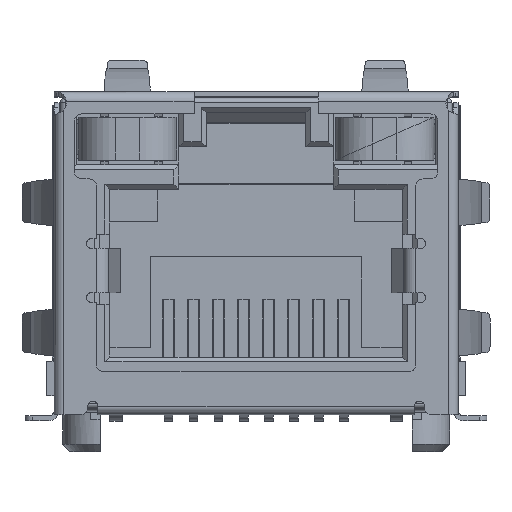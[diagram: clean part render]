
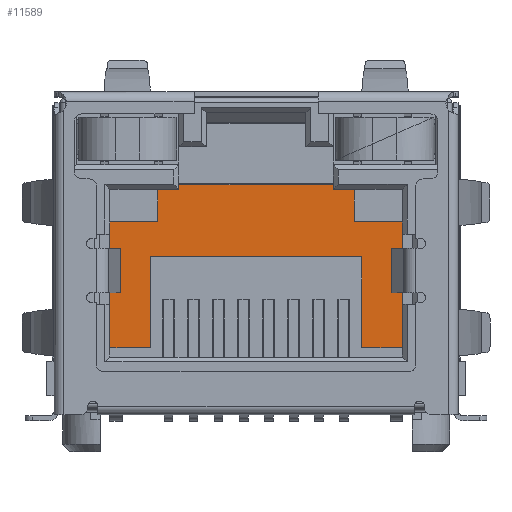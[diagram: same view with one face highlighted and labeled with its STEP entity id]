
A CAD part, top view. The second image highlights one B-rep face of the part: STEP entity #11589.
In plain terms, the highlighted planar face has unit normal (0, 0, 1).
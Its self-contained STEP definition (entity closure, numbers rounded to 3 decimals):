
#21 = LINE ( 'NONE', #16234, #8757 ) ;
#443 = CARTESIAN_POINT ( 'NONE',  ( 12.275, 2.65, -12. ) ) ;
#582 = ORIENTED_EDGE ( 'NONE', *, *, #8021, .T. ) ;
#1001 = EDGE_CURVE ( 'NONE', #19019, #26712, #17330, .T. ) ;
#1640 = ORIENTED_EDGE ( 'NONE', *, *, #19144, .T. ) ;
#1658 = VECTOR ( 'NONE', #27479, 1000. ) ;
#2353 = VERTEX_POINT ( 'NONE', #30650 ) ;
#2451 = VECTOR ( 'NONE', #25251, 1000. ) ;
#2607 = CARTESIAN_POINT ( 'NONE',  ( 11.975, 9.08, -12. ) ) ;
#2632 = DIRECTION ( 'NONE',  ( 1., 0., 0. ) ) ;
#2642 = CARTESIAN_POINT ( 'NONE',  ( 3.975, 9.08, -12. ) ) ;
#3118 = VERTEX_POINT ( 'NONE', #12124 ) ;
#3523 = CARTESIAN_POINT ( 'NONE',  ( 4.825, 9.28, -12. ) ) ;
#3684 = CARTESIAN_POINT ( 'NONE',  ( 3.675, 6.35, -12. ) ) ;
#4426 = VECTOR ( 'NONE', #23660, 1000. ) ;
#4626 = VECTOR ( 'NONE', #25375, 1000. ) ;
#4784 = CARTESIAN_POINT ( 'NONE',  ( 3.975, 9.08, -12. ) ) ;
#5159 = CARTESIAN_POINT ( 'NONE',  ( 3.975, 7.78, -12. ) ) ;
#5240 = VECTOR ( 'NONE', #17037, 1000. ) ;
#5432 = CARTESIAN_POINT ( 'NONE',  ( 13.93, 2.65, -12. ) ) ;
#5595 = CARTESIAN_POINT ( 'NONE',  ( 13.93, 9.08, -12. ) ) ;
#6303 = VECTOR ( 'NONE', #30928, 1000. ) ;
#6496 = CARTESIAN_POINT ( 'NONE',  ( 2.02, 9.08, -12. ) ) ;
#6897 = CARTESIAN_POINT ( 'NONE',  ( 2.02, 2.25, -12. ) ) ;
#7446 = VECTOR ( 'NONE', #9847, 1000. ) ;
#7973 = VERTEX_POINT ( 'NONE', #12334 ) ;
#8021 = EDGE_CURVE ( 'NONE', #22386, #17427, #24111, .T. ) ;
#8704 = EDGE_CURVE ( 'NONE', #9073, #27555, #12447, .T. ) ;
#8757 = VECTOR ( 'NONE', #15993, 1000. ) ;
#9073 = VERTEX_POINT ( 'NONE', #20763 ) ;
#9608 = EDGE_CURVE ( 'NONE', #26712, #19454, #23378, .T. ) ;
#9847 = DIRECTION ( 'NONE',  ( 0., -1., 0. ) ) ;
#9963 = CARTESIAN_POINT ( 'NONE',  ( 12.275, 2.45, -12. ) ) ;
#10271 = CARTESIAN_POINT ( 'NONE',  ( 3.675, 2.65, -12. ) ) ;
#10468 = CARTESIAN_POINT ( 'NONE',  ( 2.02, 2.65, -12. ) ) ;
#10705 = DIRECTION ( 'NONE',  ( 0., -1., 0. ) ) ;
#10788 = LINE ( 'NONE', #23855, #29496 ) ;
#11002 = CARTESIAN_POINT ( 'NONE',  ( 11.125, 9.08, -12. ) ) ;
#11055 = LINE ( 'NONE', #12738, #4426 ) ;
#11277 = LINE ( 'NONE', #14454, #16670 ) ;
#11494 = LINE ( 'NONE', #5595, #29804 ) ;
#11589 = ADVANCED_FACE ( 'NONE', ( #12782 ), #23865, .T. ) ;
#11652 = ORIENTED_EDGE ( 'NONE', *, *, #27666, .T. ) ;
#12124 = CARTESIAN_POINT ( 'NONE',  ( 4.825, 9.08, -12. ) ) ;
#12257 = ORIENTED_EDGE ( 'NONE', *, *, #17317, .T. ) ;
#12334 = CARTESIAN_POINT ( 'NONE',  ( 11.975, 7.78, -12. ) ) ;
#12447 = LINE ( 'NONE', #3523, #31194 ) ;
#12451 = CARTESIAN_POINT ( 'NONE',  ( 2.02, 2.65, -12. ) ) ;
#12486 = LINE ( 'NONE', #6897, #6303 ) ;
#12537 = VECTOR ( 'NONE', #26985, 1000. ) ;
#12738 = CARTESIAN_POINT ( 'NONE',  ( 2.02, 9.08, -12. ) ) ;
#12782 = FACE_OUTER_BOUND ( 'NONE', #18361, .T. ) ;
#12788 = LINE ( 'NONE', #9963, #7446 ) ;
#12811 = AXIS2_PLACEMENT_3D ( 'NONE', #28884, #18516, #2632 ) ;
#13929 = VECTOR ( 'NONE', #22245, 1000. ) ;
#14320 = CARTESIAN_POINT ( 'NONE',  ( 4.825, 9.28, -12. ) ) ;
#14323 = ORIENTED_EDGE ( 'NONE', *, *, #19095, .T. ) ;
#14454 = CARTESIAN_POINT ( 'NONE',  ( 11.975, 7.78, -12. ) ) ;
#14729 = DIRECTION ( 'NONE',  ( 0., 1., 0. ) ) ;
#15052 = VERTEX_POINT ( 'NONE', #3684 ) ;
#15258 = VECTOR ( 'NONE', #15535, 1000. ) ;
#15332 = VERTEX_POINT ( 'NONE', #2607 ) ;
#15535 = DIRECTION ( 'NONE',  ( 0., -1., 0. ) ) ;
#15618 = DIRECTION ( 'NONE',  ( 0., -1., 0. ) ) ;
#15724 = CARTESIAN_POINT ( 'NONE',  ( 2.02, 7.78, -12. ) ) ;
#15993 = DIRECTION ( 'NONE',  ( -1., 0., 0. ) ) ;
#15996 = LINE ( 'NONE', #30656, #5240 ) ;
#16234 = CARTESIAN_POINT ( 'NONE',  ( 13.93, 2.65, -12. ) ) ;
#16390 = VERTEX_POINT ( 'NONE', #443 ) ;
#16482 = EDGE_CURVE ( 'NONE', #24926, #16390, #21, .T. ) ;
#16670 = VECTOR ( 'NONE', #22248, 1000. ) ;
#16799 = ORIENTED_EDGE ( 'NONE', *, *, #18976, .T. ) ;
#16865 = EDGE_CURVE ( 'NONE', #27555, #3118, #10788, .T. ) ;
#17037 = DIRECTION ( 'NONE',  ( 1., 0., 0. ) ) ;
#17317 = EDGE_CURVE ( 'NONE', #22808, #9073, #21507, .T. ) ;
#17330 = LINE ( 'NONE', #4784, #15258 ) ;
#17427 = VERTEX_POINT ( 'NONE', #10271 ) ;
#18361 = EDGE_LOOP ( 'NONE', ( #22834, #23411, #582, #33631, #1640, #11652, #19473, #29431, #25728, #28910, #16799, #12257, #23415, #32358, #14323, #32825 ) ) ;
#18516 = DIRECTION ( 'NONE',  ( 0., 0., 1. ) ) ;
#18584 = EDGE_CURVE ( 'NONE', #2353, #24926, #11494, .T. ) ;
#18976 = EDGE_CURVE ( 'NONE', #15332, #22808, #11055, .T. ) ;
#19019 = VERTEX_POINT ( 'NONE', #2642 ) ;
#19095 = EDGE_CURVE ( 'NONE', #3118, #19019, #33505, .T. ) ;
#19144 = EDGE_CURVE ( 'NONE', #15052, #28843, #15996, .T. ) ;
#19454 = VERTEX_POINT ( 'NONE', #15724 ) ;
#19473 = ORIENTED_EDGE ( 'NONE', *, *, #16482, .F. ) ;
#19544 = CARTESIAN_POINT ( 'NONE',  ( 2.02, 7.78, -12. ) ) ;
#20742 = CARTESIAN_POINT ( 'NONE',  ( 12.275, 6.35, -12. ) ) ;
#20763 = CARTESIAN_POINT ( 'NONE',  ( 11.125, 9.28, -12. ) ) ;
#21507 = LINE ( 'NONE', #22673, #2451 ) ;
#21615 = DIRECTION ( 'NONE',  ( -1., 0., 0. ) ) ;
#22245 = DIRECTION ( 'NONE',  ( -1., 0., 0. ) ) ;
#22248 = DIRECTION ( 'NONE',  ( 0., 1., 0. ) ) ;
#22386 = VERTEX_POINT ( 'NONE', #10468 ) ;
#22673 = CARTESIAN_POINT ( 'NONE',  ( 11.125, 2.45, -12. ) ) ;
#22808 = VERTEX_POINT ( 'NONE', #11002 ) ;
#22834 = ORIENTED_EDGE ( 'NONE', *, *, #9608, .T. ) ;
#23378 = LINE ( 'NONE', #27463, #12537 ) ;
#23411 = ORIENTED_EDGE ( 'NONE', *, *, #25609, .F. ) ;
#23415 = ORIENTED_EDGE ( 'NONE', *, *, #8704, .T. ) ;
#23660 = DIRECTION ( 'NONE',  ( -1., 0., 0. ) ) ;
#23855 = CARTESIAN_POINT ( 'NONE',  ( 4.825, 2.45, -12. ) ) ;
#23865 = PLANE ( 'NONE',  #12811 ) ;
#24111 = LINE ( 'NONE', #12451, #4626 ) ;
#24926 = VERTEX_POINT ( 'NONE', #5432 ) ;
#24946 = LINE ( 'NONE', #19544, #1658 ) ;
#25251 = DIRECTION ( 'NONE',  ( 0., 1., 0. ) ) ;
#25375 = DIRECTION ( 'NONE',  ( 1., 0., 0. ) ) ;
#25609 = EDGE_CURVE ( 'NONE', #22386, #19454, #12486, .T. ) ;
#25728 = ORIENTED_EDGE ( 'NONE', *, *, #31307, .T. ) ;
#26109 = EDGE_CURVE ( 'NONE', #7973, #15332, #11277, .T. ) ;
#26712 = VERTEX_POINT ( 'NONE', #5159 ) ;
#26985 = DIRECTION ( 'NONE',  ( -1., 0., 0. ) ) ;
#27463 = CARTESIAN_POINT ( 'NONE',  ( 2.02, 7.78, -12. ) ) ;
#27479 = DIRECTION ( 'NONE',  ( -1., 0., 0. ) ) ;
#27555 = VERTEX_POINT ( 'NONE', #14320 ) ;
#27666 = EDGE_CURVE ( 'NONE', #28843, #16390, #12788, .T. ) ;
#28130 = CARTESIAN_POINT ( 'NONE',  ( 3.675, 2.45, -12. ) ) ;
#28761 = EDGE_CURVE ( 'NONE', #17427, #15052, #33126, .T. ) ;
#28843 = VERTEX_POINT ( 'NONE', #20742 ) ;
#28884 = CARTESIAN_POINT ( 'NONE',  ( 2.02, 2.45, -12. ) ) ;
#28910 = ORIENTED_EDGE ( 'NONE', *, *, #26109, .T. ) ;
#29431 = ORIENTED_EDGE ( 'NONE', *, *, #18584, .F. ) ;
#29496 = VECTOR ( 'NONE', #15618, 1000. ) ;
#29804 = VECTOR ( 'NONE', #10705, 1000. ) ;
#30636 = VECTOR ( 'NONE', #14729, 1000. ) ;
#30650 = CARTESIAN_POINT ( 'NONE',  ( 13.93, 7.78, -12. ) ) ;
#30656 = CARTESIAN_POINT ( 'NONE',  ( 2.02, 6.35, -12. ) ) ;
#30928 = DIRECTION ( 'NONE',  ( 0., 1., 0. ) ) ;
#31194 = VECTOR ( 'NONE', #21615, 1000. ) ;
#31307 = EDGE_CURVE ( 'NONE', #2353, #7973, #24946, .T. ) ;
#32358 = ORIENTED_EDGE ( 'NONE', *, *, #16865, .T. ) ;
#32825 = ORIENTED_EDGE ( 'NONE', *, *, #1001, .T. ) ;
#33126 = LINE ( 'NONE', #28130, #30636 ) ;
#33505 = LINE ( 'NONE', #6496, #13929 ) ;
#33631 = ORIENTED_EDGE ( 'NONE', *, *, #28761, .T. ) ;
